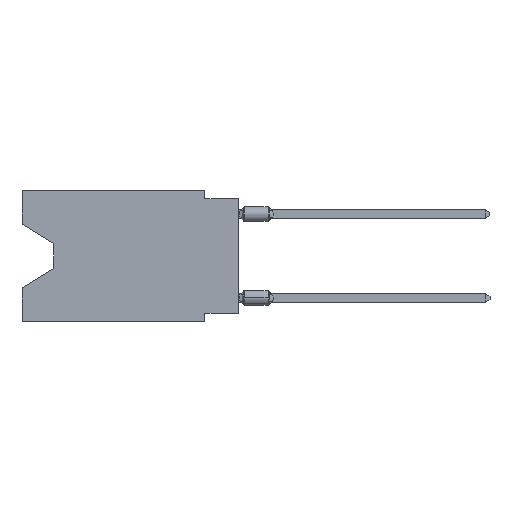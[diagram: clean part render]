
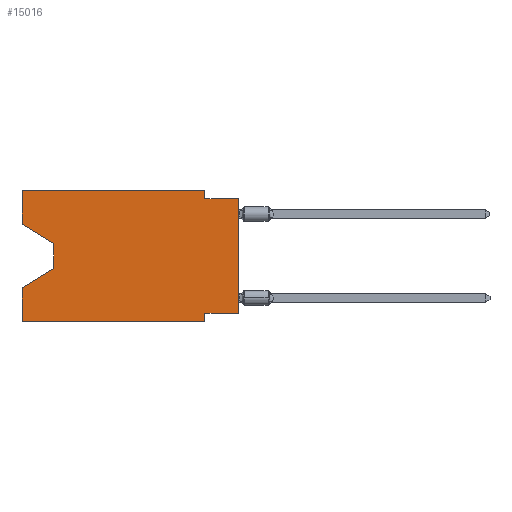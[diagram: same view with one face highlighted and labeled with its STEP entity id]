
A CAD part, left-side view. The second image highlights one B-rep face of the part: STEP entity #15016.
In plain terms, the highlighted planar face has unit normal (-1, 0, 0).
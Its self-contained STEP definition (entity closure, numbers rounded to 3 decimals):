
#347 = EDGE_CURVE ( 'NONE', #1773, #14471, #14517, .T. ) ;
#506 = EDGE_CURVE ( 'NONE', #11224, #9521, #1894, .T. ) ;
#515 = DIRECTION ( 'NONE',  ( 0., 0., -1. ) ) ;
#600 = ORIENTED_EDGE ( 'NONE', *, *, #8218, .F. ) ;
#796 = CARTESIAN_POINT ( 'NONE',  ( 0., 16.383, -7.36 ) ) ;
#1259 = ORIENTED_EDGE ( 'NONE', *, *, #14550, .T. ) ;
#1287 = DIRECTION ( 'NONE',  ( 0., 0., -1. ) ) ;
#1369 = VECTOR ( 'NONE', #12889, 1000. ) ;
#1538 = DIRECTION ( 'NONE',  ( 0., 0., 1. ) ) ;
#1689 = EDGE_CURVE ( 'NONE', #9403, #15615, #6328, .T. ) ;
#1724 = DIRECTION ( 'NONE',  ( 0., 0., 1. ) ) ;
#1749 = CARTESIAN_POINT ( 'NONE',  ( 0., 16.383, -9.906 ) ) ;
#1773 = VERTEX_POINT ( 'NONE', #8932 ) ;
#1780 = VECTOR ( 'NONE', #9437, 1000. ) ;
#1894 = LINE ( 'NONE', #11459, #4428 ) ;
#1950 = CARTESIAN_POINT ( 'NONE',  ( 0., 0., 0. ) ) ;
#2039 = EDGE_CURVE ( 'NONE', #9403, #7031, #13840, .T. ) ;
#2159 = ORIENTED_EDGE ( 'NONE', *, *, #10911, .T. ) ;
#2222 = CARTESIAN_POINT ( 'NONE',  ( 0., 16.383, 0. ) ) ;
#2264 = CARTESIAN_POINT ( 'NONE',  ( 0., 2.54, -0.635 ) ) ;
#2387 = ORIENTED_EDGE ( 'NONE', *, *, #2039, .T. ) ;
#2537 = FACE_OUTER_BOUND ( 'NONE', #12546, .T. ) ;
#2614 = DIRECTION ( 'NONE',  ( 0., -1., 0. ) ) ;
#2933 = AXIS2_PLACEMENT_3D ( 'NONE', #7071, #5071, #515 ) ;
#3049 = LINE ( 'NONE', #11559, #13935 ) ;
#3559 = CARTESIAN_POINT ( 'NONE',  ( 0., 13.97, -5.893 ) ) ;
#3592 = CARTESIAN_POINT ( 'NONE',  ( 0., 16.383, -2.546 ) ) ;
#3672 = LINE ( 'NONE', #6082, #14707 ) ;
#3769 = CARTESIAN_POINT ( 'NONE',  ( 0., 2.54, -9.906 ) ) ;
#3940 = ORIENTED_EDGE ( 'NONE', *, *, #1689, .F. ) ;
#4239 = DIRECTION ( 'NONE',  ( 0., -1., 0. ) ) ;
#4255 = LINE ( 'NONE', #1950, #7312 ) ;
#4428 = VECTOR ( 'NONE', #12905, 1000. ) ;
#5071 = DIRECTION ( 'NONE',  ( 1., 0., 0. ) ) ;
#5300 = EDGE_CURVE ( 'NONE', #11224, #13807, #4255, .T. ) ;
#5314 = CARTESIAN_POINT ( 'NONE',  ( 0., 2.54, -9.271 ) ) ;
#5317 = ORIENTED_EDGE ( 'NONE', *, *, #5624, .F. ) ;
#5597 = DIRECTION ( 'NONE',  ( 0., 0., 1. ) ) ;
#5624 = EDGE_CURVE ( 'NONE', #14191, #13807, #3049, .T. ) ;
#5828 = EDGE_CURVE ( 'NONE', #10668, #14191, #3672, .T. ) ;
#6082 = CARTESIAN_POINT ( 'NONE',  ( 0., 2.54, 0. ) ) ;
#6315 = ORIENTED_EDGE ( 'NONE', *, *, #5300, .T. ) ;
#6328 = LINE ( 'NONE', #12141, #12360 ) ;
#6447 = CARTESIAN_POINT ( 'NONE',  ( 0., 16.383, -9.906 ) ) ;
#6711 = VECTOR ( 'NONE', #1287, 1000. ) ;
#6831 = CARTESIAN_POINT ( 'NONE',  ( 0., 13.97, -4.013 ) ) ;
#6974 = VECTOR ( 'NONE', #14563, 1000. ) ;
#6990 = VECTOR ( 'NONE', #1724, 1000. ) ;
#6994 = ORIENTED_EDGE ( 'NONE', *, *, #15031, .F. ) ;
#7031 = VERTEX_POINT ( 'NONE', #13414 ) ;
#7071 = CARTESIAN_POINT ( 'NONE',  ( 0., 16.383, 0. ) ) ;
#7148 = CARTESIAN_POINT ( 'NONE',  ( 0., 13.97, -4.013 ) ) ;
#7312 = VECTOR ( 'NONE', #5597, 1000. ) ;
#7346 = LINE ( 'NONE', #3769, #6711 ) ;
#7936 = ORIENTED_EDGE ( 'NONE', *, *, #14297, .F. ) ;
#8170 = DIRECTION ( 'NONE',  ( 0., -1., 0. ) ) ;
#8218 = EDGE_CURVE ( 'NONE', #9885, #10668, #15535, .T. ) ;
#8564 = CARTESIAN_POINT ( 'NONE',  ( 0., 16.383, 0. ) ) ;
#8590 = ORIENTED_EDGE ( 'NONE', *, *, #347, .T. ) ;
#8932 = CARTESIAN_POINT ( 'NONE',  ( 0., 16.383, -2.546 ) ) ;
#9355 = CARTESIAN_POINT ( 'NONE',  ( 0., 0., -0.635 ) ) ;
#9403 = VERTEX_POINT ( 'NONE', #1749 ) ;
#9437 = DIRECTION ( 'NONE',  ( 0., 0.855, -0.519 ) ) ;
#9521 = VERTEX_POINT ( 'NONE', #5314 ) ;
#9612 = VECTOR ( 'NONE', #8170, 1000. ) ;
#9885 = VERTEX_POINT ( 'NONE', #8564 ) ;
#10023 = CARTESIAN_POINT ( 'NONE',  ( 0., 13.97, -5.893 ) ) ;
#10668 = VERTEX_POINT ( 'NONE', #13313 ) ;
#10729 = LINE ( 'NONE', #7148, #6974 ) ;
#10911 = EDGE_CURVE ( 'NONE', #11821, #15615, #15594, .T. ) ;
#11169 = DIRECTION ( 'NONE',  ( 0., 0., -1. ) ) ;
#11224 = VERTEX_POINT ( 'NONE', #15398 ) ;
#11435 = CARTESIAN_POINT ( 'NONE',  ( 0., 16.383, 0. ) ) ;
#11459 = CARTESIAN_POINT ( 'NONE',  ( 0., 0., -9.271 ) ) ;
#11559 = CARTESIAN_POINT ( 'NONE',  ( 0., 0., -0.635 ) ) ;
#11821 = VERTEX_POINT ( 'NONE', #10023 ) ;
#12141 = CARTESIAN_POINT ( 'NONE',  ( 0., 16.383, 0. ) ) ;
#12246 = PLANE ( 'NONE',  #2933 ) ;
#12360 = VECTOR ( 'NONE', #1538, 1000. ) ;
#12546 = EDGE_LOOP ( 'NONE', ( #8590, #1259, #2159, #3940, #2387, #7936, #14656, #6315, #5317, #12570, #600, #6994 ) ) ;
#12570 = ORIENTED_EDGE ( 'NONE', *, *, #5828, .F. ) ;
#12889 = DIRECTION ( 'NONE',  ( 0., -0.855, -0.519 ) ) ;
#12905 = DIRECTION ( 'NONE',  ( 0., 1., 0. ) ) ;
#13313 = CARTESIAN_POINT ( 'NONE',  ( 0., 2.54, 0. ) ) ;
#13414 = CARTESIAN_POINT ( 'NONE',  ( 0., 2.54, -9.906 ) ) ;
#13807 = VERTEX_POINT ( 'NONE', #9355 ) ;
#13840 = LINE ( 'NONE', #6447, #15169 ) ;
#13935 = VECTOR ( 'NONE', #4239, 1000. ) ;
#14191 = VERTEX_POINT ( 'NONE', #2264 ) ;
#14297 = EDGE_CURVE ( 'NONE', #9521, #7031, #7346, .T. ) ;
#14471 = VERTEX_POINT ( 'NONE', #6831 ) ;
#14517 = LINE ( 'NONE', #3592, #1369 ) ;
#14550 = EDGE_CURVE ( 'NONE', #14471, #11821, #10729, .T. ) ;
#14563 = DIRECTION ( 'NONE',  ( 0., 0., -1. ) ) ;
#14656 = ORIENTED_EDGE ( 'NONE', *, *, #506, .F. ) ;
#14707 = VECTOR ( 'NONE', #11169, 1000. ) ;
#14805 = LINE ( 'NONE', #11435, #6990 ) ;
#15016 = ADVANCED_FACE ( 'NONE', ( #2537 ), #12246, .F. ) ;
#15031 = EDGE_CURVE ( 'NONE', #1773, #9885, #14805, .T. ) ;
#15169 = VECTOR ( 'NONE', #2614, 1000. ) ;
#15398 = CARTESIAN_POINT ( 'NONE',  ( 0., 0., -9.271 ) ) ;
#15535 = LINE ( 'NONE', #2222, #9612 ) ;
#15594 = LINE ( 'NONE', #3559, #1780 ) ;
#15615 = VERTEX_POINT ( 'NONE', #796 ) ;
